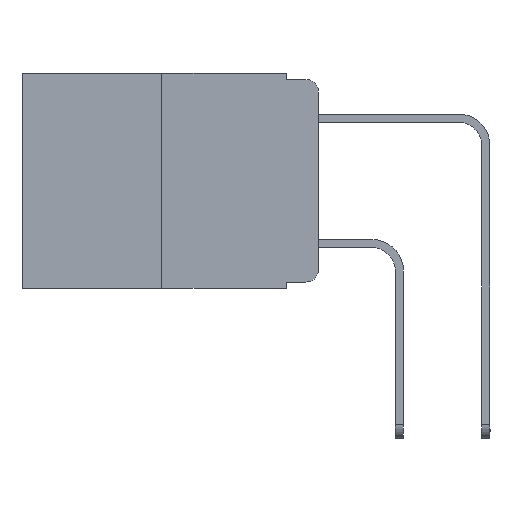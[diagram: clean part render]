
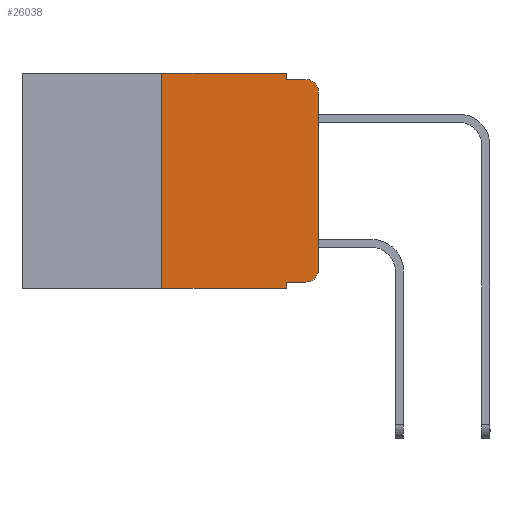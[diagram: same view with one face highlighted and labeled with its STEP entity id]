
A CAD part, left-side view. The second image highlights one B-rep face of the part: STEP entity #26038.
In plain terms, the highlighted planar face has unit normal (-1, 0, 0).
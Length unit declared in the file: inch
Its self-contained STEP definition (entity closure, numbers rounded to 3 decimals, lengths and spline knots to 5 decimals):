
#867 = VECTOR ( 'NONE', #11795, 39.37008 ) ;
#1410 = VERTEX_POINT ( 'NONE', #5177 ) ;
#1714 = ORIENTED_EDGE ( 'NONE', *, *, #12728, .T. ) ;
#1765 = VECTOR ( 'NONE', #26338, 39.37008 ) ;
#2441 = DIRECTION ( 'NONE',  ( 0., 0., -1. ) ) ;
#2524 = CARTESIAN_POINT ( 'NONE',  ( 0., 0.051, -0.343 ) ) ;
#2679 = EDGE_LOOP ( 'NONE', ( #7670, #1714, #12302, #5781, #2963, #16891, #5489, #22278, #24729, #21979 ) ) ;
#2722 = DIRECTION ( 'NONE',  ( 1., 0., 0. ) ) ;
#2963 = ORIENTED_EDGE ( 'NONE', *, *, #9658, .F. ) ;
#3171 = CIRCLE ( 'NONE', #20308, 0.02 ) ;
#3204 = VERTEX_POINT ( 'NONE', #16577 ) ;
#3976 = AXIS2_PLACEMENT_3D ( 'NONE', #6250, #26305, #12039 ) ;
#5177 = CARTESIAN_POINT ( 'NONE',  ( 0., 0.051, -0.333 ) ) ;
#5358 = CARTESIAN_POINT ( 'NONE',  ( 0., 0.25, 0. ) ) ;
#5489 = ORIENTED_EDGE ( 'NONE', *, *, #19486, .T. ) ;
#5781 = ORIENTED_EDGE ( 'NONE', *, *, #10157, .F. ) ;
#6250 = CARTESIAN_POINT ( 'NONE',  ( 0., 0.02, -0.03 ) ) ;
#7026 = CARTESIAN_POINT ( 'NONE',  ( 0., 0.051, 0. ) ) ;
#7134 = VERTEX_POINT ( 'NONE', #8073 ) ;
#7670 = ORIENTED_EDGE ( 'NONE', *, *, #23935, .T. ) ;
#8073 = CARTESIAN_POINT ( 'NONE',  ( 0., 0.02, -0.333 ) ) ;
#8165 = CARTESIAN_POINT ( 'NONE',  ( 0., 0., 0. ) ) ;
#8577 = VERTEX_POINT ( 'NONE', #9887 ) ;
#8626 = VERTEX_POINT ( 'NONE', #5358 ) ;
#8739 = FACE_OUTER_BOUND ( 'NONE', #2679, .T. ) ;
#8870 = CARTESIAN_POINT ( 'NONE',  ( 0., 0.02, -0.01 ) ) ;
#9032 = DIRECTION ( 'NONE',  ( 0., 0., -1. ) ) ;
#9141 = DIRECTION ( 'NONE',  ( 0., -1., 0. ) ) ;
#9182 = DIRECTION ( 'NONE',  ( 0., -1., 0. ) ) ;
#9585 = CARTESIAN_POINT ( 'NONE',  ( 0., 0.051, 0. ) ) ;
#9658 = EDGE_CURVE ( 'NONE', #8626, #21525, #15463, .T. ) ;
#9887 = CARTESIAN_POINT ( 'NONE',  ( 0., 0., -0.313 ) ) ;
#10079 = VECTOR ( 'NONE', #9032, 39.37008 ) ;
#10157 = EDGE_CURVE ( 'NONE', #21525, #16228, #22757, .T. ) ;
#11795 = DIRECTION ( 'NONE',  ( 0., 0., -1. ) ) ;
#12039 = DIRECTION ( 'NONE',  ( 0., 0., -1. ) ) ;
#12302 = ORIENTED_EDGE ( 'NONE', *, *, #23897, .F. ) ;
#12327 = CARTESIAN_POINT ( 'NONE',  ( 0., 0.051, -0.01 ) ) ;
#12728 = EDGE_CURVE ( 'NONE', #24338, #26030, #26296, .T. ) ;
#14090 = DIRECTION ( 'NONE',  ( 0., 0., 1. ) ) ;
#14364 = DIRECTION ( 'NONE',  ( 0., 0., -1. ) ) ;
#14926 = PLANE ( 'NONE',  #21145 ) ;
#15463 = LINE ( 'NONE', #19641, #23587 ) ;
#15627 = CARTESIAN_POINT ( 'NONE',  ( 0., 0.25, 0. ) ) ;
#15646 = VECTOR ( 'NONE', #9182, 39.37008 ) ;
#15891 = LINE ( 'NONE', #23568, #17082 ) ;
#15997 = VECTOR ( 'NONE', #21934, 39.37008 ) ;
#16099 = EDGE_CURVE ( 'NONE', #1410, #7134, #19940, .T. ) ;
#16228 = VERTEX_POINT ( 'NONE', #16871 ) ;
#16497 = LINE ( 'NONE', #8165, #22782 ) ;
#16577 = CARTESIAN_POINT ( 'NONE',  ( 0., 0.25, -0.343 ) ) ;
#16730 = EDGE_CURVE ( 'NONE', #1410, #20865, #21535, .T. ) ;
#16871 = CARTESIAN_POINT ( 'NONE',  ( 0., 0.051, -0.01 ) ) ;
#16891 = ORIENTED_EDGE ( 'NONE', *, *, #25741, .F. ) ;
#17082 = VECTOR ( 'NONE', #17509, 39.37008 ) ;
#17509 = DIRECTION ( 'NONE',  ( 0., -1., 0. ) ) ;
#17713 = CARTESIAN_POINT ( 'NONE',  ( 0., 0.051, 0. ) ) ;
#17905 = CARTESIAN_POINT ( 'NONE',  ( 0., 0.051, -0.333 ) ) ;
#19486 = EDGE_CURVE ( 'NONE', #3204, #20865, #15891, .T. ) ;
#19641 = CARTESIAN_POINT ( 'NONE',  ( 0., 0.473, 0. ) ) ;
#19940 = LINE ( 'NONE', #17905, #15646 ) ;
#20019 = LINE ( 'NONE', #12327, #1765 ) ;
#20308 = AXIS2_PLACEMENT_3D ( 'NONE', #26217, #26353, #14364 ) ;
#20865 = VERTEX_POINT ( 'NONE', #2524 ) ;
#21145 = AXIS2_PLACEMENT_3D ( 'NONE', #21246, #2722, #2441 ) ;
#21246 = CARTESIAN_POINT ( 'NONE',  ( 0., 0.473, 0. ) ) ;
#21525 = VERTEX_POINT ( 'NONE', #9585 ) ;
#21535 = LINE ( 'NONE', #7026, #10079 ) ;
#21934 = DIRECTION ( 'NONE',  ( 0., 0., 1. ) ) ;
#21979 = ORIENTED_EDGE ( 'NONE', *, *, #26275, .T. ) ;
#22278 = ORIENTED_EDGE ( 'NONE', *, *, #16730, .F. ) ;
#22757 = LINE ( 'NONE', #17713, #867 ) ;
#22782 = VECTOR ( 'NONE', #14090, 39.37008 ) ;
#23568 = CARTESIAN_POINT ( 'NONE',  ( 0., 0.473, -0.343 ) ) ;
#23587 = VECTOR ( 'NONE', #9141, 39.37008 ) ;
#23897 = EDGE_CURVE ( 'NONE', #16228, #26030, #20019, .T. ) ;
#23935 = EDGE_CURVE ( 'NONE', #8577, #24338, #16497, .T. ) ;
#23963 = LINE ( 'NONE', #15627, #15997 ) ;
#24153 = CARTESIAN_POINT ( 'NONE',  ( 0., 0., -0.03 ) ) ;
#24338 = VERTEX_POINT ( 'NONE', #24153 ) ;
#24729 = ORIENTED_EDGE ( 'NONE', *, *, #16099, .T. ) ;
#25741 = EDGE_CURVE ( 'NONE', #3204, #8626, #23963, .T. ) ;
#26030 = VERTEX_POINT ( 'NONE', #8870 ) ;
#26038 = ADVANCED_FACE ( 'NONE', ( #8739 ), #14926, .F. ) ;
#26217 = CARTESIAN_POINT ( 'NONE',  ( 0., 0.02, -0.313 ) ) ;
#26275 = EDGE_CURVE ( 'NONE', #7134, #8577, #3171, .T. ) ;
#26296 = CIRCLE ( 'NONE', #3976, 0.02 ) ;
#26305 = DIRECTION ( 'NONE',  ( -1., 0., 0. ) ) ;
#26338 = DIRECTION ( 'NONE',  ( 0., -1., 0. ) ) ;
#26353 = DIRECTION ( 'NONE',  ( -1., 0., 0. ) ) ;
